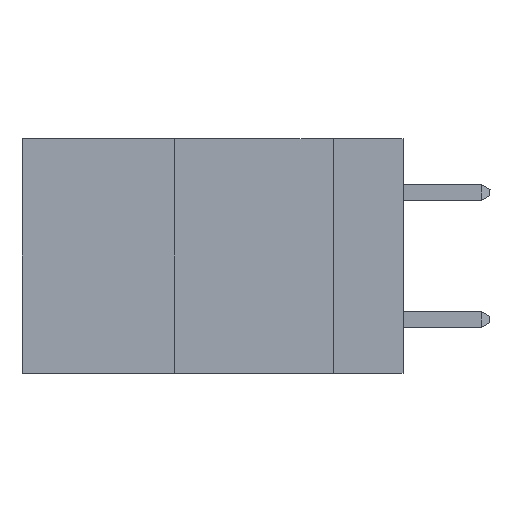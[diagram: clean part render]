
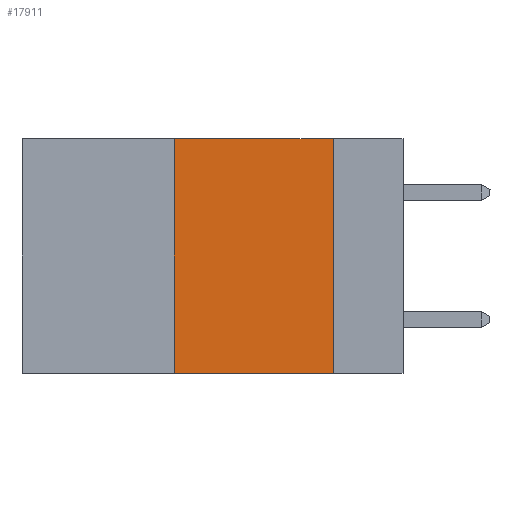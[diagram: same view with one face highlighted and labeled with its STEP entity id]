
A CAD part, left-side view. The second image highlights one B-rep face of the part: STEP entity #17911.
In plain terms, the highlighted planar face has unit normal (-1, 0, 0).
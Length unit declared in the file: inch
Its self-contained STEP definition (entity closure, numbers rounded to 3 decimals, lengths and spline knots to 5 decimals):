
#953 = EDGE_CURVE ( 'NONE', #14923, #3117, #17740, .T. ) ;
#1463 = CARTESIAN_POINT ( 'NONE',  ( 0., 0.6, 0. ) ) ;
#1580 = VECTOR ( 'NONE', #14054, 39.37008 ) ;
#2244 = VERTEX_POINT ( 'NONE', #5934 ) ;
#3117 = VERTEX_POINT ( 'NONE', #17738 ) ;
#3261 = ORIENTED_EDGE ( 'NONE', *, *, #5308, .F. ) ;
#4406 = PLANE ( 'NONE',  #14986 ) ;
#4482 = VECTOR ( 'NONE', #10112, 39.37008 ) ;
#5308 = EDGE_CURVE ( 'NONE', #14923, #2244, #5430, .T. ) ;
#5421 = EDGE_CURVE ( 'NONE', #2244, #10548, #12453, .T. ) ;
#5430 = LINE ( 'NONE', #6754, #4482 ) ;
#5934 = CARTESIAN_POINT ( 'NONE',  ( 0., 0.36, 0. ) ) ;
#6116 = DIRECTION ( 'NONE',  ( 0., -1., 0. ) ) ;
#6671 = CARTESIAN_POINT ( 'NONE',  ( 0., 0.11, 0. ) ) ;
#6754 = CARTESIAN_POINT ( 'NONE',  ( 0., 0.36, 0. ) ) ;
#7268 = VECTOR ( 'NONE', #6116, 39.37008 ) ;
#8516 = CARTESIAN_POINT ( 'NONE',  ( 0., 0.6, 0. ) ) ;
#9282 = CARTESIAN_POINT ( 'NONE',  ( 0., 0.6, -0.37 ) ) ;
#10065 = FACE_OUTER_BOUND ( 'NONE', #11261, .T. ) ;
#10112 = DIRECTION ( 'NONE',  ( 0., 0., 1. ) ) ;
#10141 = VECTOR ( 'NONE', #11977, 39.37008 ) ;
#10548 = VERTEX_POINT ( 'NONE', #13020 ) ;
#11261 = EDGE_LOOP ( 'NONE', ( #18001, #14892, #3261, #18548 ) ) ;
#11307 = CARTESIAN_POINT ( 'NONE',  ( 0., 0.36, -0.37 ) ) ;
#11977 = DIRECTION ( 'NONE',  ( 0., -1., 0. ) ) ;
#12366 = LINE ( 'NONE', #6671, #1580 ) ;
#12453 = LINE ( 'NONE', #8516, #10141 ) ;
#13020 = CARTESIAN_POINT ( 'NONE',  ( 0., 0.11, 0. ) ) ;
#14054 = DIRECTION ( 'NONE',  ( 0., 0., -1. ) ) ;
#14892 = ORIENTED_EDGE ( 'NONE', *, *, #5421, .F. ) ;
#14897 = DIRECTION ( 'NONE',  ( 1., 0., 0. ) ) ;
#14923 = VERTEX_POINT ( 'NONE', #11307 ) ;
#14986 = AXIS2_PLACEMENT_3D ( 'NONE', #1463, #14897, #15005 ) ;
#15005 = DIRECTION ( 'NONE',  ( 0., 0., -1. ) ) ;
#17738 = CARTESIAN_POINT ( 'NONE',  ( 0., 0.11, -0.37 ) ) ;
#17740 = LINE ( 'NONE', #9282, #7268 ) ;
#17911 = ADVANCED_FACE ( 'NONE', ( #10065 ), #4406, .F. ) ;
#18001 = ORIENTED_EDGE ( 'NONE', *, *, #18444, .F. ) ;
#18444 = EDGE_CURVE ( 'NONE', #10548, #3117, #12366, .T. ) ;
#18548 = ORIENTED_EDGE ( 'NONE', *, *, #953, .T. ) ;
